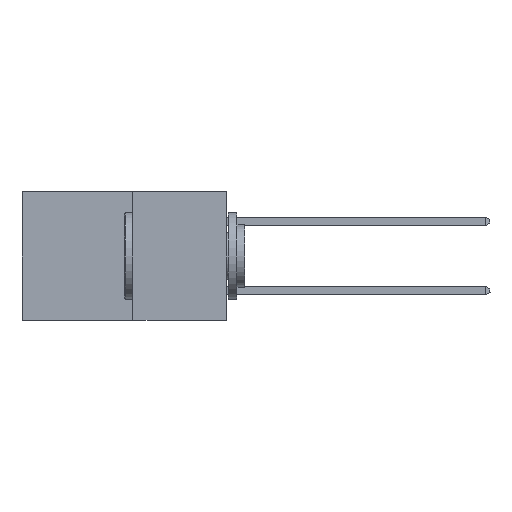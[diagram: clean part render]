
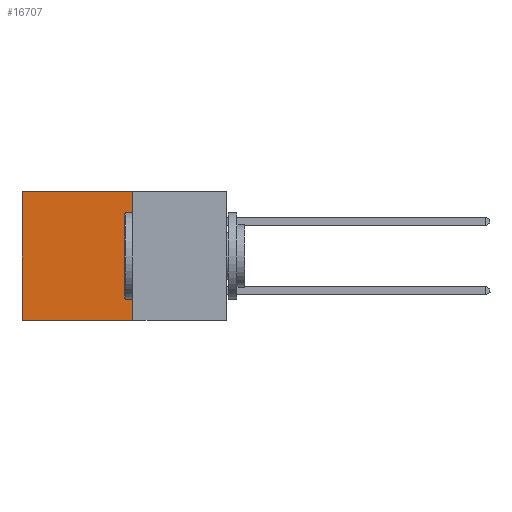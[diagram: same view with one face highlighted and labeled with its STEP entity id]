
A CAD part, left-side view. The second image highlights one B-rep face of the part: STEP entity #16707.
In plain terms, the highlighted planar face has unit normal (-1, 0, 0).
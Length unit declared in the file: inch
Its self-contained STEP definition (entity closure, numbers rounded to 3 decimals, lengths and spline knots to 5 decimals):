
#1797 = VECTOR ( 'NONE', #8392, 39.37008 ) ;
#1974 = DIRECTION ( 'NONE',  ( 0., 0., -1. ) ) ;
#2873 = ORIENTED_EDGE ( 'NONE', *, *, #16703, .T. ) ;
#4089 = VECTOR ( 'NONE', #7121, 39.37008 ) ;
#4164 = CARTESIAN_POINT ( 'NONE',  ( 0.277, 0.27, 0. ) ) ;
#5059 = VERTEX_POINT ( 'NONE', #10184 ) ;
#5531 = DIRECTION ( 'NONE',  ( 0., 0., -1. ) ) ;
#5612 = VERTEX_POINT ( 'NONE', #23401 ) ;
#7121 = DIRECTION ( 'NONE',  ( 0., 1., 0. ) ) ;
#8392 = DIRECTION ( 'NONE',  ( 0., 0., -1. ) ) ;
#10184 = CARTESIAN_POINT ( 'NONE',  ( 0.277, 0.27, 0. ) ) ;
#10567 = CARTESIAN_POINT ( 'NONE',  ( 0.277, 0.59, -0.37 ) ) ;
#10662 = DIRECTION ( 'NONE',  ( 0., 1., 0. ) ) ;
#10669 = AXIS2_PLACEMENT_3D ( 'NONE', #23578, #14874, #1974 ) ;
#11179 = ORIENTED_EDGE ( 'NONE', *, *, #16717, .T. ) ;
#11607 = VECTOR ( 'NONE', #5531, 39.37008 ) ;
#13257 = FACE_OUTER_BOUND ( 'NONE', #21153, .T. ) ;
#14783 = VERTEX_POINT ( 'NONE', #14923 ) ;
#14874 = DIRECTION ( 'NONE',  ( 1., 0., 0. ) ) ;
#14923 = CARTESIAN_POINT ( 'NONE',  ( 0.277, 0.27, -0.37 ) ) ;
#15711 = EDGE_CURVE ( 'NONE', #5059, #14783, #23180, .T. ) ;
#16703 = EDGE_CURVE ( 'NONE', #5612, #19684, #24885, .T. ) ;
#16707 = ADVANCED_FACE ( 'NONE', ( #13257 ), #27927, .F. ) ;
#16717 = EDGE_CURVE ( 'NONE', #5059, #5612, #18338, .T. ) ;
#17649 = VECTOR ( 'NONE', #10662, 39.37008 ) ;
#18338 = LINE ( 'NONE', #4164, #17649 ) ;
#19676 = CARTESIAN_POINT ( 'NONE',  ( 0.277, 0.59, -0.37 ) ) ;
#19684 = VERTEX_POINT ( 'NONE', #19676 ) ;
#20079 = CARTESIAN_POINT ( 'NONE',  ( 0.277, 0.27, -0.37 ) ) ;
#20645 = CARTESIAN_POINT ( 'NONE',  ( 0.277, 0.27, -0.37 ) ) ;
#20648 = LINE ( 'NONE', #20079, #4089 ) ;
#21153 = EDGE_LOOP ( 'NONE', ( #2873, #22200, #26465, #11179 ) ) ;
#22200 = ORIENTED_EDGE ( 'NONE', *, *, #26764, .F. ) ;
#23180 = LINE ( 'NONE', #20645, #11607 ) ;
#23401 = CARTESIAN_POINT ( 'NONE',  ( 0.277, 0.59, 0. ) ) ;
#23578 = CARTESIAN_POINT ( 'NONE',  ( 0.277, 0.27, -0.37 ) ) ;
#24885 = LINE ( 'NONE', #10567, #1797 ) ;
#26465 = ORIENTED_EDGE ( 'NONE', *, *, #15711, .F. ) ;
#26764 = EDGE_CURVE ( 'NONE', #14783, #19684, #20648, .T. ) ;
#27927 = PLANE ( 'NONE',  #10669 ) ;
